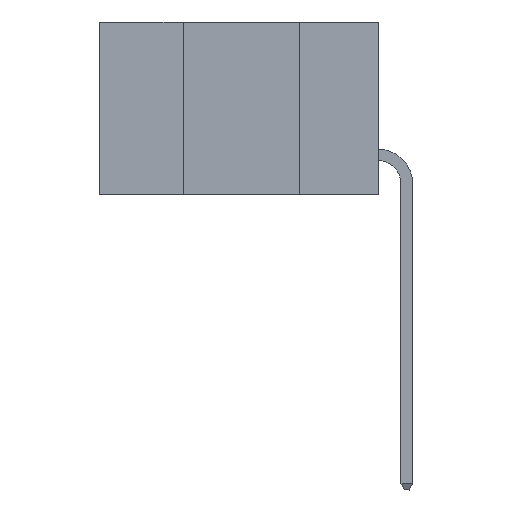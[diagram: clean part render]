
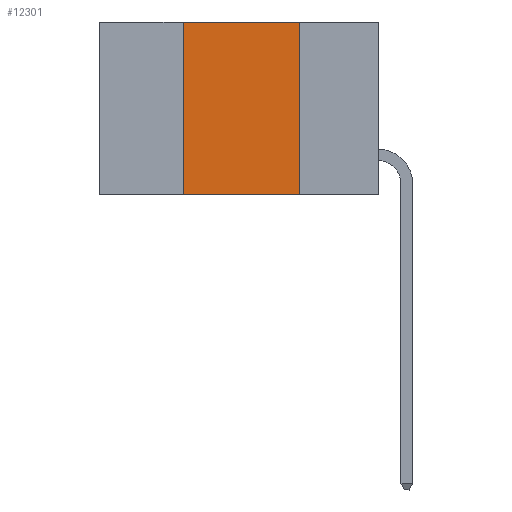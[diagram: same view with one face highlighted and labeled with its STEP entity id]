
A CAD part, left-side view. The second image highlights one B-rep face of the part: STEP entity #12301.
In plain terms, the highlighted planar face has unit normal (-1, 0, 0).
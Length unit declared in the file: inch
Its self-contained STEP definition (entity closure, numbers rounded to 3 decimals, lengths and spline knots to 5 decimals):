
#2 = VECTOR ( 'NONE', #596, 39.37008 ) ;
#199 = FACE_OUTER_BOUND ( 'NONE', #8288, .T. ) ;
#315 = VERTEX_POINT ( 'NONE', #14014 ) ;
#413 = ORIENTED_EDGE ( 'NONE', *, *, #5500, .F. ) ;
#596 = DIRECTION ( 'NONE',  ( 0., 0., 1. ) ) ;
#740 = LINE ( 'NONE', #3055, #5028 ) ;
#819 = DIRECTION ( 'NONE',  ( 0., 0., -1. ) ) ;
#1559 = LINE ( 'NONE', #9773, #14802 ) ;
#2043 = ORIENTED_EDGE ( 'NONE', *, *, #14151, .T. ) ;
#2142 = EDGE_CURVE ( 'NONE', #2404, #13674, #740, .T. ) ;
#2404 = VERTEX_POINT ( 'NONE', #12070 ) ;
#2405 = ORIENTED_EDGE ( 'NONE', *, *, #2142, .F. ) ;
#2416 = CARTESIAN_POINT ( 'NONE',  ( 0., 0.6, 0. ) ) ;
#3055 = CARTESIAN_POINT ( 'NONE',  ( 0., 0.17, -0.37 ) ) ;
#4751 = LINE ( 'NONE', #2416, #5712 ) ;
#4814 = DIRECTION ( 'NONE',  ( 1., 0., 0. ) ) ;
#4877 = AXIS2_PLACEMENT_3D ( 'NONE', #8020, #4814, #12861 ) ;
#4902 = ORIENTED_EDGE ( 'NONE', *, *, #8399, .F. ) ;
#5028 = VECTOR ( 'NONE', #819, 39.37008 ) ;
#5500 = EDGE_CURVE ( 'NONE', #6684, #2404, #4751, .T. ) ;
#5712 = VECTOR ( 'NONE', #9355, 39.37008 ) ;
#6068 = PLANE ( 'NONE',  #4877 ) ;
#6238 = LINE ( 'NONE', #9576, #2 ) ;
#6684 = VERTEX_POINT ( 'NONE', #7296 ) ;
#7296 = CARTESIAN_POINT ( 'NONE',  ( 0., 0.42, 0. ) ) ;
#8020 = CARTESIAN_POINT ( 'NONE',  ( 0., 0.6, 0. ) ) ;
#8288 = EDGE_LOOP ( 'NONE', ( #2405, #413, #4902, #2043 ) ) ;
#8399 = EDGE_CURVE ( 'NONE', #315, #6684, #6238, .T. ) ;
#9355 = DIRECTION ( 'NONE',  ( 0., -1., 0. ) ) ;
#9430 = CARTESIAN_POINT ( 'NONE',  ( 0., 0.17, -0.37 ) ) ;
#9576 = CARTESIAN_POINT ( 'NONE',  ( 0., 0.42, -0.37 ) ) ;
#9773 = CARTESIAN_POINT ( 'NONE',  ( 0., 0.6, -0.37 ) ) ;
#12014 = DIRECTION ( 'NONE',  ( 0., -1., 0. ) ) ;
#12070 = CARTESIAN_POINT ( 'NONE',  ( 0., 0.17, 0. ) ) ;
#12301 = ADVANCED_FACE ( 'NONE', ( #199 ), #6068, .F. ) ;
#12861 = DIRECTION ( 'NONE',  ( 0., 0., -1. ) ) ;
#13674 = VERTEX_POINT ( 'NONE', #9430 ) ;
#14014 = CARTESIAN_POINT ( 'NONE',  ( 0., 0.42, -0.37 ) ) ;
#14151 = EDGE_CURVE ( 'NONE', #315, #13674, #1559, .T. ) ;
#14802 = VECTOR ( 'NONE', #12014, 39.37008 ) ;
